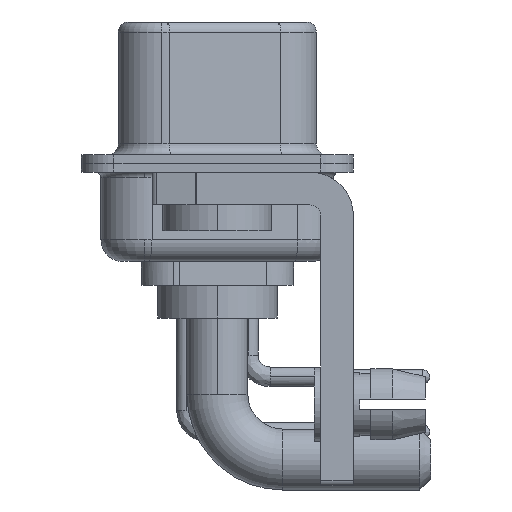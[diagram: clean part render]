
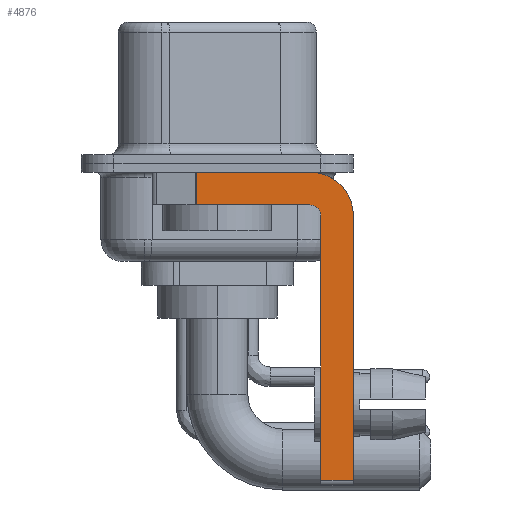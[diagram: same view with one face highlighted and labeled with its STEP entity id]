
A CAD part, left-side view. The second image highlights one B-rep face of the part: STEP entity #4876.
In plain terms, the highlighted planar face has unit normal (-1, 0, 0).
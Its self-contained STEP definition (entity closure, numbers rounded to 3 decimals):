
#80 = ORIENTED_EDGE ( 'NONE', *, *, #18701, .F. ) ;
#295 = CIRCLE ( 'NONE', #22601, 0.5 ) ;
#707 = VECTOR ( 'NONE', #17453, 1000. ) ;
#772 = LINE ( 'NONE', #26347, #707 ) ;
#1159 = VERTEX_POINT ( 'NONE', #17091 ) ;
#1560 = VERTEX_POINT ( 'NONE', #6544 ) ;
#1636 = ORIENTED_EDGE ( 'NONE', *, *, #2727, .F. ) ;
#1778 = DIRECTION ( 'NONE',  ( -1., 0., 0. ) ) ;
#1864 = CIRCLE ( 'NONE', #18909, 2. ) ;
#2606 = LINE ( 'NONE', #6229, #18600 ) ;
#2727 = EDGE_CURVE ( 'NONE', #20346, #1560, #295, .T. ) ;
#2960 = DIRECTION ( 'NONE',  ( 0., -1., 0. ) ) ;
#2961 = VECTOR ( 'NONE', #24930, 1000. ) ;
#3726 = EDGE_CURVE ( 'NONE', #20245, #1159, #2606, .T. ) ;
#4697 = ORIENTED_EDGE ( 'NONE', *, *, #19020, .F. ) ;
#4788 = DIRECTION ( 'NONE',  ( 0., -1., 0. ) ) ;
#4833 = LINE ( 'NONE', #26039, #13253 ) ;
#4863 = ORIENTED_EDGE ( 'NONE', *, *, #3726, .F. ) ;
#4876 = ADVANCED_FACE ( 'NONE', ( #23418 ), #6461, .F. ) ;
#5244 = ORIENTED_EDGE ( 'NONE', *, *, #9013, .F. ) ;
#5863 = CARTESIAN_POINT ( 'NONE',  ( -2.9, -4.25, -2.4 ) ) ;
#6229 = CARTESIAN_POINT ( 'NONE',  ( -2.9, 3., -0.4 ) ) ;
#6253 = EDGE_CURVE ( 'NONE', #11087, #19349, #17733, .T. ) ;
#6461 = PLANE ( 'NONE',  #6680 ) ;
#6480 = CARTESIAN_POINT ( 'NONE',  ( -2.9, 0.978, -1.9 ) ) ;
#6544 = CARTESIAN_POINT ( 'NONE',  ( -2.9, -4.25, -1.9 ) ) ;
#6680 = AXIS2_PLACEMENT_3D ( 'NONE', #21383, #15210, #25077 ) ;
#6980 = VERTEX_POINT ( 'NONE', #18056 ) ;
#7307 = DIRECTION ( 'NONE',  ( 0., 0., -1. ) ) ;
#7417 = DIRECTION ( 'NONE',  ( 0., 0., -1. ) ) ;
#8124 = CARTESIAN_POINT ( 'NONE',  ( -2.9, -4.75, -14.8 ) ) ;
#8213 = DIRECTION ( 'NONE',  ( 0., 0., 1. ) ) ;
#8883 = CARTESIAN_POINT ( 'NONE',  ( -2.9, -6.25, -14.55 ) ) ;
#9013 = EDGE_CURVE ( 'NONE', #1560, #12179, #772, .T. ) ;
#10847 = EDGE_CURVE ( 'NONE', #20245, #12179, #14666, .T. ) ;
#11087 = VERTEX_POINT ( 'NONE', #26675 ) ;
#11276 = CARTESIAN_POINT ( 'NONE',  ( -2.9, 0.978, -0.4 ) ) ;
#12058 = CARTESIAN_POINT ( 'NONE',  ( -2.9, -4.25, -2.4 ) ) ;
#12179 = VERTEX_POINT ( 'NONE', #6480 ) ;
#13253 = VECTOR ( 'NONE', #7307, 1000. ) ;
#13335 = CARTESIAN_POINT ( 'NONE',  ( -2.9, -4.75, -2.4 ) ) ;
#14666 = LINE ( 'NONE', #18381, #2961 ) ;
#15210 = DIRECTION ( 'NONE',  ( 1., 0., 0. ) ) ;
#17091 = CARTESIAN_POINT ( 'NONE',  ( -2.9, -4.25, -0.4 ) ) ;
#17453 = DIRECTION ( 'NONE',  ( 0., 1., 0. ) ) ;
#17733 = LINE ( 'NONE', #21456, #23763 ) ;
#18056 = CARTESIAN_POINT ( 'NONE',  ( -2.9, -6.25, -2.4 ) ) ;
#18381 = CARTESIAN_POINT ( 'NONE',  ( -2.9, 0.978, -1.9 ) ) ;
#18446 = EDGE_CURVE ( 'NONE', #6980, #19349, #4833, .T. ) ;
#18532 = LINE ( 'NONE', #8124, #23703 ) ;
#18600 = VECTOR ( 'NONE', #4788, 1000. ) ;
#18701 = EDGE_CURVE ( 'NONE', #11087, #20346, #18532, .T. ) ;
#18909 = AXIS2_PLACEMENT_3D ( 'NONE', #12058, #24516, #7417 ) ;
#19020 = EDGE_CURVE ( 'NONE', #1159, #6980, #1864, .T. ) ;
#19349 = VERTEX_POINT ( 'NONE', #8883 ) ;
#20245 = VERTEX_POINT ( 'NONE', #11276 ) ;
#20346 = VERTEX_POINT ( 'NONE', #13335 ) ;
#20396 = ORIENTED_EDGE ( 'NONE', *, *, #6253, .T. ) ;
#20559 = ORIENTED_EDGE ( 'NONE', *, *, #18446, .F. ) ;
#21383 = CARTESIAN_POINT ( 'NONE',  ( -2.9, -4.25, -2.4 ) ) ;
#21456 = CARTESIAN_POINT ( 'NONE',  ( -2.9, -4.25, -14.55 ) ) ;
#22601 = AXIS2_PLACEMENT_3D ( 'NONE', #5863, #1778, #8213 ) ;
#23418 = FACE_OUTER_BOUND ( 'NONE', #23485, .T. ) ;
#23485 = EDGE_LOOP ( 'NONE', ( #4863, #26388, #5244, #1636, #80, #20396, #20559, #4697 ) ) ;
#23703 = VECTOR ( 'NONE', #27013, 1000. ) ;
#23763 = VECTOR ( 'NONE', #2960, 1000. ) ;
#24516 = DIRECTION ( 'NONE',  ( 1., 0., 0. ) ) ;
#24930 = DIRECTION ( 'NONE',  ( 0., 0., -1. ) ) ;
#25077 = DIRECTION ( 'NONE',  ( 0., 0., -1. ) ) ;
#26039 = CARTESIAN_POINT ( 'NONE',  ( -2.9, -6.25, -2.4 ) ) ;
#26347 = CARTESIAN_POINT ( 'NONE',  ( -2.9, -4.25, -1.9 ) ) ;
#26388 = ORIENTED_EDGE ( 'NONE', *, *, #10847, .T. ) ;
#26675 = CARTESIAN_POINT ( 'NONE',  ( -2.9, -4.75, -14.55 ) ) ;
#27013 = DIRECTION ( 'NONE',  ( 0., 0., 1. ) ) ;
